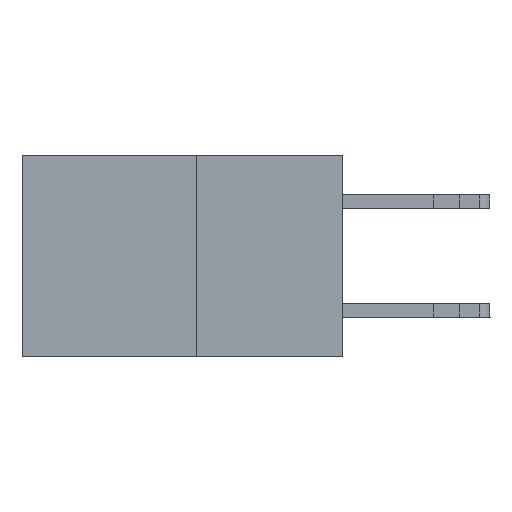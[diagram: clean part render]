
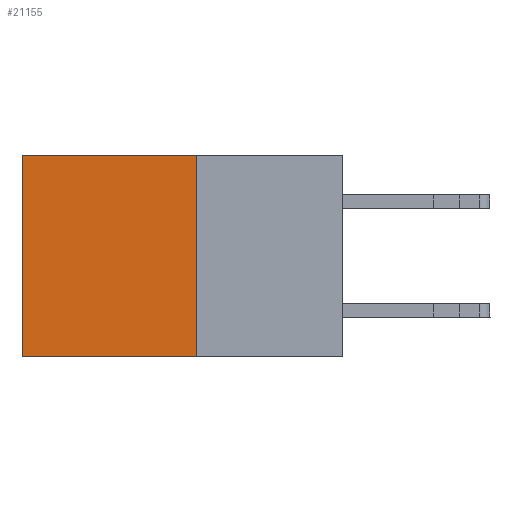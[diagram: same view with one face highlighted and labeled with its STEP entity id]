
A CAD part, left-side view. The second image highlights one B-rep face of the part: STEP entity #21155.
In plain terms, the highlighted planar face has unit normal (-1, 0, 0).
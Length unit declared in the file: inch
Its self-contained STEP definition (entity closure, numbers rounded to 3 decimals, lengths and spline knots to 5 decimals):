
#379 = VERTEX_POINT ( 'NONE', #10427 ) ;
#1384 = VECTOR ( 'NONE', #4072, 39.37008 ) ;
#1415 = DIRECTION ( 'NONE',  ( 0., 0., -1. ) ) ;
#1817 = EDGE_CURVE ( 'NONE', #19115, #379, #14694, .T. ) ;
#1984 = LINE ( 'NONE', #2166, #1384 ) ;
#2166 = CARTESIAN_POINT ( 'NONE',  ( 0.277, 0.27, -0.37 ) ) ;
#2282 = CARTESIAN_POINT ( 'NONE',  ( 0.277, 0.27, -0.37 ) ) ;
#2363 = DIRECTION ( 'NONE',  ( 0., 0., -1. ) ) ;
#3153 = CARTESIAN_POINT ( 'NONE',  ( 0.277, 0.27, 0. ) ) ;
#4072 = DIRECTION ( 'NONE',  ( 0., 0., -1. ) ) ;
#4239 = EDGE_LOOP ( 'NONE', ( #4306, #14251, #5497, #13467 ) ) ;
#4306 = ORIENTED_EDGE ( 'NONE', *, *, #1817, .T. ) ;
#4674 = AXIS2_PLACEMENT_3D ( 'NONE', #6975, #12243, #1415 ) ;
#5299 = CARTESIAN_POINT ( 'NONE',  ( 0.277, 0.59, -0.37 ) ) ;
#5497 = ORIENTED_EDGE ( 'NONE', *, *, #17587, .F. ) ;
#6975 = CARTESIAN_POINT ( 'NONE',  ( 0.277, 0.27, -0.37 ) ) ;
#7092 = DIRECTION ( 'NONE',  ( 0., 1., 0. ) ) ;
#9409 = VERTEX_POINT ( 'NONE', #3153 ) ;
#10090 = FACE_OUTER_BOUND ( 'NONE', #4239, .T. ) ;
#10427 = CARTESIAN_POINT ( 'NONE',  ( 0.277, 0.59, -0.37 ) ) ;
#10488 = PLANE ( 'NONE',  #4674 ) ;
#10499 = VERTEX_POINT ( 'NONE', #2282 ) ;
#12170 = CARTESIAN_POINT ( 'NONE',  ( 0.277, 0.59, 0. ) ) ;
#12243 = DIRECTION ( 'NONE',  ( 1., 0., 0. ) ) ;
#12279 = CARTESIAN_POINT ( 'NONE',  ( 0.277, 0.27, 0. ) ) ;
#13191 = CARTESIAN_POINT ( 'NONE',  ( 0.277, 0.27, -0.37 ) ) ;
#13467 = ORIENTED_EDGE ( 'NONE', *, *, #18523, .T. ) ;
#14251 = ORIENTED_EDGE ( 'NONE', *, *, #20158, .F. ) ;
#14470 = LINE ( 'NONE', #13191, #17362 ) ;
#14694 = LINE ( 'NONE', #5299, #19191 ) ;
#14915 = DIRECTION ( 'NONE',  ( 0., 1., 0. ) ) ;
#16136 = LINE ( 'NONE', #12279, #20122 ) ;
#17362 = VECTOR ( 'NONE', #14915, 39.37008 ) ;
#17587 = EDGE_CURVE ( 'NONE', #9409, #10499, #1984, .T. ) ;
#18523 = EDGE_CURVE ( 'NONE', #9409, #19115, #16136, .T. ) ;
#19115 = VERTEX_POINT ( 'NONE', #12170 ) ;
#19191 = VECTOR ( 'NONE', #2363, 39.37008 ) ;
#20122 = VECTOR ( 'NONE', #7092, 39.37008 ) ;
#20158 = EDGE_CURVE ( 'NONE', #10499, #379, #14470, .T. ) ;
#21155 = ADVANCED_FACE ( 'NONE', ( #10090 ), #10488, .F. ) ;
